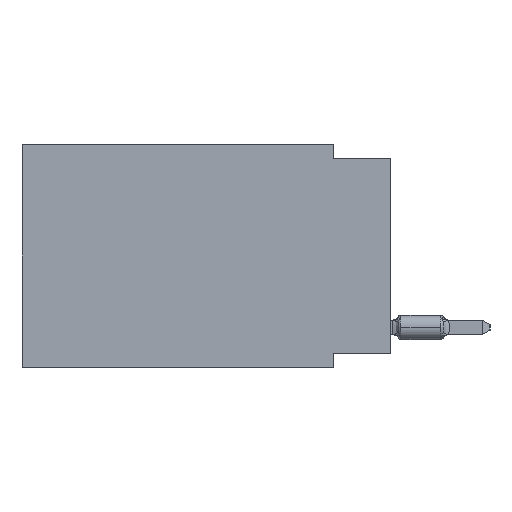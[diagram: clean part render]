
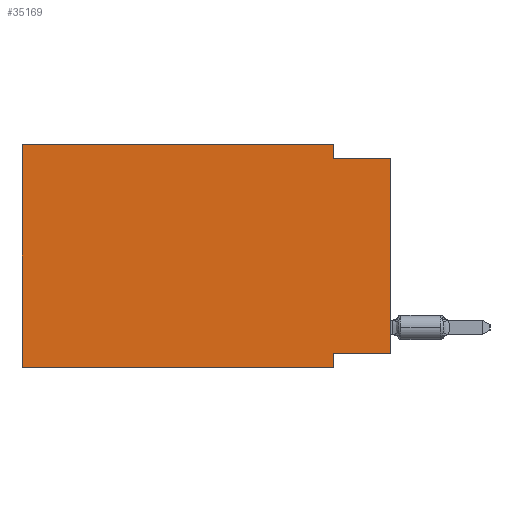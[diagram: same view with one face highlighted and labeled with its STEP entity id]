
A CAD part, left-side view. The second image highlights one B-rep face of the part: STEP entity #35169.
In plain terms, the highlighted planar face has unit normal (-1, 0, 0).
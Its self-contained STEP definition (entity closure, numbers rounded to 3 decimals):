
#348 = LINE ( 'NONE', #25244, #14944 ) ;
#1207 = LINE ( 'NONE', #1585, #60087 ) ;
#1547 = PLANE ( 'NONE',  #14104 ) ;
#1585 = CARTESIAN_POINT ( 'NONE',  ( 0., 0., 0. ) ) ;
#2023 = EDGE_CURVE ( 'NONE', #69648, #43532, #52295, .T. ) ;
#3329 = LINE ( 'NONE', #14085, #32974 ) ;
#5897 = EDGE_CURVE ( 'NONE', #14696, #11089, #348, .T. ) ;
#7053 = CARTESIAN_POINT ( 'NONE',  ( 0., 0., -0.635 ) ) ;
#7211 = VECTOR ( 'NONE', #17422, 1000. ) ;
#8003 = EDGE_CURVE ( 'NONE', #19234, #26142, #18174, .T. ) ;
#11089 = VERTEX_POINT ( 'NONE', #23163 ) ;
#13036 = ORIENTED_EDGE ( 'NONE', *, *, #16547, .F. ) ;
#13808 = CARTESIAN_POINT ( 'NONE',  ( 0., 16.383, 0. ) ) ;
#14085 = CARTESIAN_POINT ( 'NONE',  ( 0., 16.383, 0. ) ) ;
#14104 = AXIS2_PLACEMENT_3D ( 'NONE', #13808, #30294, #36436 ) ;
#14123 = VECTOR ( 'NONE', #71830, 1000. ) ;
#14190 = FACE_OUTER_BOUND ( 'NONE', #35601, .T. ) ;
#14696 = VERTEX_POINT ( 'NONE', #18160 ) ;
#14826 = CARTESIAN_POINT ( 'NONE',  ( 0., 0., -0.635 ) ) ;
#14944 = VECTOR ( 'NONE', #48610, 1000. ) ;
#16287 = DIRECTION ( 'NONE',  ( 0., -1., 0. ) ) ;
#16547 = EDGE_CURVE ( 'NONE', #11089, #19234, #74038, .T. ) ;
#17286 = VECTOR ( 'NONE', #16287, 1000. ) ;
#17422 = DIRECTION ( 'NONE',  ( 0., 1., 0. ) ) ;
#18160 = CARTESIAN_POINT ( 'NONE',  ( 0., 16.383, 0. ) ) ;
#18174 = LINE ( 'NONE', #7053, #14123 ) ;
#18797 = VECTOR ( 'NONE', #45916, 1000. ) ;
#19234 = VERTEX_POINT ( 'NONE', #31169 ) ;
#20016 = CARTESIAN_POINT ( 'NONE',  ( 0., 16.383, -9.906 ) ) ;
#21525 = CARTESIAN_POINT ( 'NONE',  ( 0., 2.54, 0. ) ) ;
#23163 = CARTESIAN_POINT ( 'NONE',  ( 0., 2.54, 0. ) ) ;
#23738 = EDGE_CURVE ( 'NONE', #69648, #26142, #1207, .T. ) ;
#24601 = ORIENTED_EDGE ( 'NONE', *, *, #2023, .F. ) ;
#25244 = CARTESIAN_POINT ( 'NONE',  ( 0., 16.383, 0. ) ) ;
#26142 = VERTEX_POINT ( 'NONE', #14826 ) ;
#28082 = ORIENTED_EDGE ( 'NONE', *, *, #5897, .F. ) ;
#29170 = VERTEX_POINT ( 'NONE', #20016 ) ;
#29740 = CARTESIAN_POINT ( 'NONE',  ( 0., 0., -9.271 ) ) ;
#30294 = DIRECTION ( 'NONE',  ( 1., 0., 0. ) ) ;
#31169 = CARTESIAN_POINT ( 'NONE',  ( 0., 2.54, -0.635 ) ) ;
#32974 = VECTOR ( 'NONE', #61189, 1000. ) ;
#35169 = ADVANCED_FACE ( 'NONE', ( #14190 ), #1547, .F. ) ;
#35601 = EDGE_LOOP ( 'NONE', ( #66346, #55514, #13036, #28082, #45313, #53899, #37129, #24601 ) ) ;
#36436 = DIRECTION ( 'NONE',  ( 0., 0., -1. ) ) ;
#37129 = ORIENTED_EDGE ( 'NONE', *, *, #44922, .F. ) ;
#42070 = VECTOR ( 'NONE', #57156, 1000. ) ;
#43532 = VERTEX_POINT ( 'NONE', #60326 ) ;
#44268 = CARTESIAN_POINT ( 'NONE',  ( 0., 16.383, -9.906 ) ) ;
#44922 = EDGE_CURVE ( 'NONE', #43532, #68021, #45523, .T. ) ;
#45313 = ORIENTED_EDGE ( 'NONE', *, *, #60185, .F. ) ;
#45397 = CARTESIAN_POINT ( 'NONE',  ( 0., 0., -9.271 ) ) ;
#45523 = LINE ( 'NONE', #68187, #18797 ) ;
#45916 = DIRECTION ( 'NONE',  ( 0., 0., -1. ) ) ;
#47696 = EDGE_CURVE ( 'NONE', #29170, #68021, #57287, .T. ) ;
#48610 = DIRECTION ( 'NONE',  ( 0., -1., 0. ) ) ;
#52295 = LINE ( 'NONE', #45397, #7211 ) ;
#53899 = ORIENTED_EDGE ( 'NONE', *, *, #47696, .T. ) ;
#55514 = ORIENTED_EDGE ( 'NONE', *, *, #8003, .F. ) ;
#57156 = DIRECTION ( 'NONE',  ( 0., 0., -1. ) ) ;
#57287 = LINE ( 'NONE', #44268, #17286 ) ;
#60087 = VECTOR ( 'NONE', #65612, 1000. ) ;
#60185 = EDGE_CURVE ( 'NONE', #29170, #14696, #3329, .T. ) ;
#60326 = CARTESIAN_POINT ( 'NONE',  ( 0., 2.54, -9.271 ) ) ;
#61189 = DIRECTION ( 'NONE',  ( 0., 0., 1. ) ) ;
#65612 = DIRECTION ( 'NONE',  ( 0., 0., 1. ) ) ;
#66346 = ORIENTED_EDGE ( 'NONE', *, *, #23738, .T. ) ;
#68021 = VERTEX_POINT ( 'NONE', #73948 ) ;
#68187 = CARTESIAN_POINT ( 'NONE',  ( 0., 2.54, -9.906 ) ) ;
#69648 = VERTEX_POINT ( 'NONE', #29740 ) ;
#71830 = DIRECTION ( 'NONE',  ( 0., -1., 0. ) ) ;
#73948 = CARTESIAN_POINT ( 'NONE',  ( 0., 2.54, -9.906 ) ) ;
#74038 = LINE ( 'NONE', #21525, #42070 ) ;
